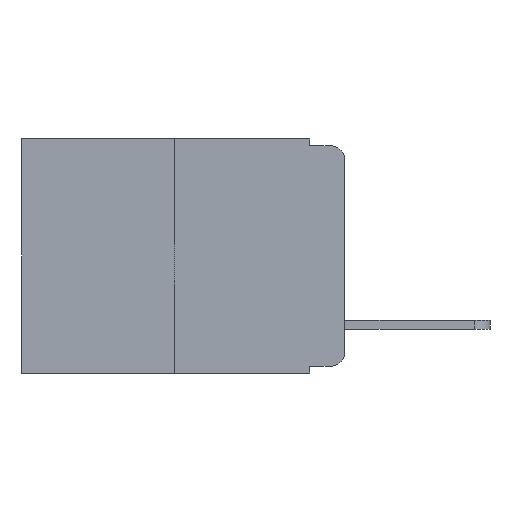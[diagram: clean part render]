
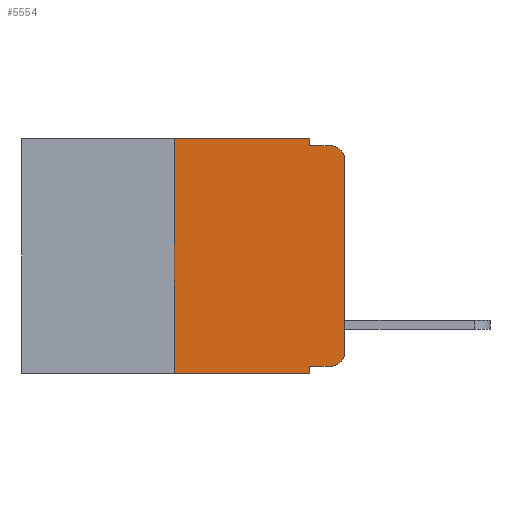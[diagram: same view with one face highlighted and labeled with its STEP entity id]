
A CAD part, left-side view. The second image highlights one B-rep face of the part: STEP entity #5554.
In plain terms, the highlighted planar face has unit normal (-1, 0, 0).
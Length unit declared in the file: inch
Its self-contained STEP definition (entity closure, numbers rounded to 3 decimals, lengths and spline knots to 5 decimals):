
#751 = CARTESIAN_POINT ( 'NONE',  ( 0., 0.473, 0. ) ) ;
#786 = VERTEX_POINT ( 'NONE', #18604 ) ;
#984 = VERTEX_POINT ( 'NONE', #17810 ) ;
#1297 = LINE ( 'NONE', #14230, #16707 ) ;
#1476 = EDGE_CURVE ( 'NONE', #17534, #984, #14997, .T. ) ;
#2236 = VECTOR ( 'NONE', #7594, 39.37008 ) ;
#2247 = ORIENTED_EDGE ( 'NONE', *, *, #17651, .T. ) ;
#2364 = FACE_OUTER_BOUND ( 'NONE', #5185, .T. ) ;
#2490 = EDGE_CURVE ( 'NONE', #8638, #17534, #12319, .T. ) ;
#2584 = EDGE_CURVE ( 'NONE', #786, #5607, #11319, .T. ) ;
#3404 = CARTESIAN_POINT ( 'NONE',  ( 0., 0.051, 0. ) ) ;
#3715 = DIRECTION ( 'NONE',  ( 0., -1., 0. ) ) ;
#3785 = DIRECTION ( 'NONE',  ( 0., 0., -1. ) ) ;
#4011 = ORIENTED_EDGE ( 'NONE', *, *, #11631, .T. ) ;
#4570 = CARTESIAN_POINT ( 'NONE',  ( 0., 0.02, -0.03 ) ) ;
#5010 = CARTESIAN_POINT ( 'NONE',  ( 0., 0.051, -0.333 ) ) ;
#5164 = CARTESIAN_POINT ( 'NONE',  ( 0., 0.473, 0. ) ) ;
#5185 = EDGE_LOOP ( 'NONE', ( #10239, #4011, #17644, #19451, #7472, #7323, #18977, #16811, #16772, #2247 ) ) ;
#5437 = AXIS2_PLACEMENT_3D ( 'NONE', #5164, #6993, #19624 ) ;
#5554 = ADVANCED_FACE ( 'NONE', ( #2364 ), #14544, .F. ) ;
#5590 = LINE ( 'NONE', #12820, #10785 ) ;
#5607 = VERTEX_POINT ( 'NONE', #11745 ) ;
#5915 = DIRECTION ( 'NONE',  ( -1., 0., 0. ) ) ;
#5959 = CARTESIAN_POINT ( 'NONE',  ( 0., 0.051, 0. ) ) ;
#6640 = VERTEX_POINT ( 'NONE', #15812 ) ;
#6993 = DIRECTION ( 'NONE',  ( 1., 0., 0. ) ) ;
#7118 = VECTOR ( 'NONE', #3785, 39.37008 ) ;
#7323 = ORIENTED_EDGE ( 'NONE', *, *, #8320, .F. ) ;
#7471 = CIRCLE ( 'NONE', #9154, 0.02 ) ;
#7472 = ORIENTED_EDGE ( 'NONE', *, *, #2490, .F. ) ;
#7594 = DIRECTION ( 'NONE',  ( 0., -1., 0. ) ) ;
#7879 = LINE ( 'NONE', #5010, #12568 ) ;
#7899 = EDGE_CURVE ( 'NONE', #6640, #10676, #15008, .T. ) ;
#8320 = EDGE_CURVE ( 'NONE', #16735, #8638, #1297, .T. ) ;
#8376 = VECTOR ( 'NONE', #11711, 39.37008 ) ;
#8638 = VERTEX_POINT ( 'NONE', #11980 ) ;
#8879 = LINE ( 'NONE', #10778, #2236 ) ;
#9104 = DIRECTION ( 'NONE',  ( 0., 0., -1. ) ) ;
#9154 = AXIS2_PLACEMENT_3D ( 'NONE', #11617, #17838, #16334 ) ;
#9301 = CARTESIAN_POINT ( 'NONE',  ( 0., 0., 0. ) ) ;
#9510 = EDGE_CURVE ( 'NONE', #16735, #5607, #5590, .T. ) ;
#10239 = ORIENTED_EDGE ( 'NONE', *, *, #7899, .T. ) ;
#10676 = VERTEX_POINT ( 'NONE', #15025 ) ;
#10778 = CARTESIAN_POINT ( 'NONE',  ( 0., 0.051, -0.01 ) ) ;
#10785 = VECTOR ( 'NONE', #14235, 39.37008 ) ;
#11319 = LINE ( 'NONE', #19385, #7118 ) ;
#11617 = CARTESIAN_POINT ( 'NONE',  ( 0., 0.02, -0.313 ) ) ;
#11631 = EDGE_CURVE ( 'NONE', #10676, #15094, #16586, .T. ) ;
#11711 = DIRECTION ( 'NONE',  ( 0., -1., 0. ) ) ;
#11745 = CARTESIAN_POINT ( 'NONE',  ( 0., 0.051, -0.343 ) ) ;
#11933 = DIRECTION ( 'NONE',  ( 0., 0., 1. ) ) ;
#11980 = CARTESIAN_POINT ( 'NONE',  ( 0., 0.25, 0. ) ) ;
#12083 = VECTOR ( 'NONE', #11933, 39.37008 ) ;
#12319 = LINE ( 'NONE', #751, #8376 ) ;
#12568 = VECTOR ( 'NONE', #3715, 39.37008 ) ;
#12820 = CARTESIAN_POINT ( 'NONE',  ( 0., 0.473, -0.343 ) ) ;
#13745 = CARTESIAN_POINT ( 'NONE',  ( 0., 0.25, -0.343 ) ) ;
#14230 = CARTESIAN_POINT ( 'NONE',  ( 0., 0.25, 0. ) ) ;
#14235 = DIRECTION ( 'NONE',  ( 0., -1., 0. ) ) ;
#14544 = PLANE ( 'NONE',  #5437 ) ;
#14756 = VECTOR ( 'NONE', #15498, 39.37008 ) ;
#14997 = LINE ( 'NONE', #5959, #14756 ) ;
#15008 = LINE ( 'NONE', #9301, #12083 ) ;
#15025 = CARTESIAN_POINT ( 'NONE',  ( 0., 0., -0.03 ) ) ;
#15094 = VERTEX_POINT ( 'NONE', #16525 ) ;
#15498 = DIRECTION ( 'NONE',  ( 0., 0., -1. ) ) ;
#15812 = CARTESIAN_POINT ( 'NONE',  ( 0., 0., -0.313 ) ) ;
#16334 = DIRECTION ( 'NONE',  ( 0., 0., -1. ) ) ;
#16525 = CARTESIAN_POINT ( 'NONE',  ( 0., 0.02, -0.01 ) ) ;
#16586 = CIRCLE ( 'NONE', #19835, 0.02 ) ;
#16707 = VECTOR ( 'NONE', #17308, 39.37008 ) ;
#16735 = VERTEX_POINT ( 'NONE', #13745 ) ;
#16772 = ORIENTED_EDGE ( 'NONE', *, *, #20213, .T. ) ;
#16811 = ORIENTED_EDGE ( 'NONE', *, *, #2584, .F. ) ;
#17308 = DIRECTION ( 'NONE',  ( 0., 0., 1. ) ) ;
#17534 = VERTEX_POINT ( 'NONE', #3404 ) ;
#17644 = ORIENTED_EDGE ( 'NONE', *, *, #19863, .F. ) ;
#17651 = EDGE_CURVE ( 'NONE', #18080, #6640, #7471, .T. ) ;
#17810 = CARTESIAN_POINT ( 'NONE',  ( 0., 0.051, -0.01 ) ) ;
#17838 = DIRECTION ( 'NONE',  ( -1., 0., 0. ) ) ;
#18080 = VERTEX_POINT ( 'NONE', #19059 ) ;
#18604 = CARTESIAN_POINT ( 'NONE',  ( 0., 0.051, -0.333 ) ) ;
#18977 = ORIENTED_EDGE ( 'NONE', *, *, #9510, .T. ) ;
#19059 = CARTESIAN_POINT ( 'NONE',  ( 0., 0.02, -0.333 ) ) ;
#19385 = CARTESIAN_POINT ( 'NONE',  ( 0., 0.051, 0. ) ) ;
#19451 = ORIENTED_EDGE ( 'NONE', *, *, #1476, .F. ) ;
#19624 = DIRECTION ( 'NONE',  ( 0., 0., -1. ) ) ;
#19835 = AXIS2_PLACEMENT_3D ( 'NONE', #4570, #5915, #9104 ) ;
#19863 = EDGE_CURVE ( 'NONE', #984, #15094, #8879, .T. ) ;
#20213 = EDGE_CURVE ( 'NONE', #786, #18080, #7879, .T. ) ;
